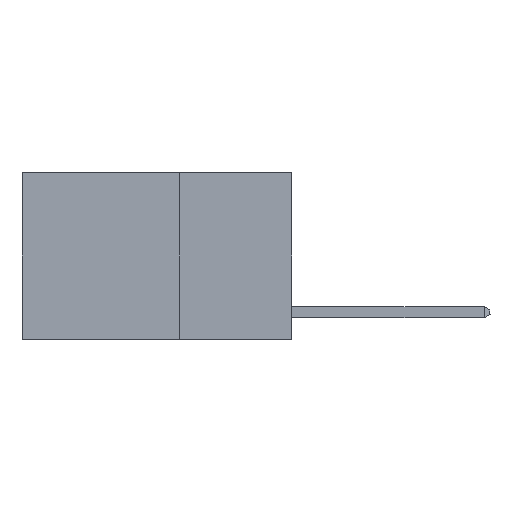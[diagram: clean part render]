
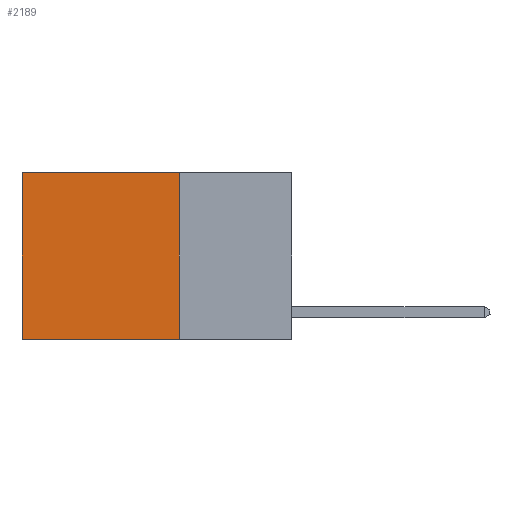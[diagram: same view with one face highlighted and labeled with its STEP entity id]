
A CAD part, left-side view. The second image highlights one B-rep face of the part: STEP entity #2189.
In plain terms, the highlighted planar face has unit normal (-1, 0, 0).
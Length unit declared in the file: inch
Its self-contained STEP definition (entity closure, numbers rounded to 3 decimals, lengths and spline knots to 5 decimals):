
#55 = PLANE ( 'NONE',  #8238 ) ;
#970 = LINE ( 'NONE', #11750, #2693 ) ;
#1749 = LINE ( 'NONE', #5822, #9914 ) ;
#2189 = ADVANCED_FACE ( 'NONE', ( #14510 ), #55, .F. ) ;
#2373 = EDGE_CURVE ( 'NONE', #19972, #3009, #6068, .T. ) ;
#2693 = VECTOR ( 'NONE', #11641, 39.37008 ) ;
#3009 = VERTEX_POINT ( 'NONE', #8802 ) ;
#4011 = ORIENTED_EDGE ( 'NONE', *, *, #14066, .F. ) ;
#4521 = EDGE_CURVE ( 'NONE', #10551, #3009, #14478, .T. ) ;
#5509 = ORIENTED_EDGE ( 'NONE', *, *, #12006, .T. ) ;
#5822 = CARTESIAN_POINT ( 'NONE',  ( 0.2625, 0.25, 0. ) ) ;
#5964 = DIRECTION ( 'NONE',  ( 0., 1., 0. ) ) ;
#6068 = LINE ( 'NONE', #11312, #22965 ) ;
#8238 = AXIS2_PLACEMENT_3D ( 'NONE', #12376, #15923, #21730 ) ;
#8802 = CARTESIAN_POINT ( 'NONE',  ( 0.2625, 0.6, -0.37 ) ) ;
#9914 = VECTOR ( 'NONE', #14433, 39.37008 ) ;
#9983 = VECTOR ( 'NONE', #18041, 39.37008 ) ;
#10551 = VERTEX_POINT ( 'NONE', #13408 ) ;
#11312 = CARTESIAN_POINT ( 'NONE',  ( 0.2625, 0.25, -0.37 ) ) ;
#11641 = DIRECTION ( 'NONE',  ( 0., 1., 0. ) ) ;
#11750 = CARTESIAN_POINT ( 'NONE',  ( 0.2625, 0.25, 0. ) ) ;
#12006 = EDGE_CURVE ( 'NONE', #17680, #10551, #970, .T. ) ;
#12376 = CARTESIAN_POINT ( 'NONE',  ( 0.2625, 0.25, 0. ) ) ;
#12702 = CARTESIAN_POINT ( 'NONE',  ( 0.2625, 0.6, 0. ) ) ;
#13408 = CARTESIAN_POINT ( 'NONE',  ( 0.2625, 0.6, 0. ) ) ;
#14066 = EDGE_CURVE ( 'NONE', #17680, #19972, #1749, .T. ) ;
#14433 = DIRECTION ( 'NONE',  ( 0., 0., -1. ) ) ;
#14478 = LINE ( 'NONE', #12702, #9983 ) ;
#14510 = FACE_OUTER_BOUND ( 'NONE', #18531, .T. ) ;
#15923 = DIRECTION ( 'NONE',  ( 1., 0., 0. ) ) ;
#17680 = VERTEX_POINT ( 'NONE', #20269 ) ;
#17689 = CARTESIAN_POINT ( 'NONE',  ( 0.2625, 0.25, -0.37 ) ) ;
#18041 = DIRECTION ( 'NONE',  ( 0., 0., -1. ) ) ;
#18531 = EDGE_LOOP ( 'NONE', ( #21177, #19627, #4011, #5509 ) ) ;
#19627 = ORIENTED_EDGE ( 'NONE', *, *, #2373, .F. ) ;
#19972 = VERTEX_POINT ( 'NONE', #17689 ) ;
#20269 = CARTESIAN_POINT ( 'NONE',  ( 0.2625, 0.25, 0. ) ) ;
#21177 = ORIENTED_EDGE ( 'NONE', *, *, #4521, .T. ) ;
#21730 = DIRECTION ( 'NONE',  ( 0., 0., -1. ) ) ;
#22965 = VECTOR ( 'NONE', #5964, 39.37008 ) ;
